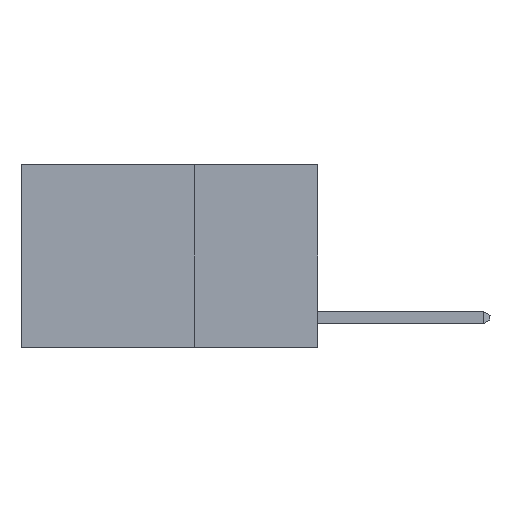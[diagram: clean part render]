
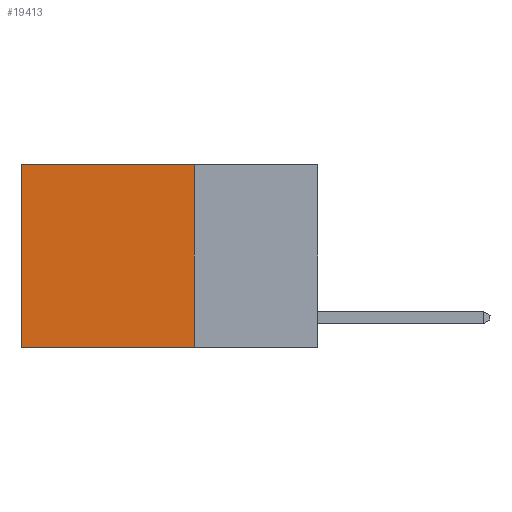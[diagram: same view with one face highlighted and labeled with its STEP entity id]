
A CAD part, left-side view. The second image highlights one B-rep face of the part: STEP entity #19413.
In plain terms, the highlighted planar face has unit normal (-1, 0, 0).
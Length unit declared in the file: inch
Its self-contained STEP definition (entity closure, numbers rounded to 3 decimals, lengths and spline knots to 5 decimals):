
#179 = ORIENTED_EDGE ( 'NONE', *, *, #16692, .T. ) ;
#418 = VECTOR ( 'NONE', #7568, 39.37008 ) ;
#4333 = PLANE ( 'NONE',  #17666 ) ;
#4831 = LINE ( 'NONE', #19243, #21026 ) ;
#5610 = CARTESIAN_POINT ( 'NONE',  ( 0.2625, 0.6, 0. ) ) ;
#5977 = DIRECTION ( 'NONE',  ( 0., 0., -1. ) ) ;
#6115 = DIRECTION ( 'NONE',  ( 0., 0., -1. ) ) ;
#6615 = ORIENTED_EDGE ( 'NONE', *, *, #10971, .F. ) ;
#6713 = VERTEX_POINT ( 'NONE', #22588 ) ;
#6715 = ORIENTED_EDGE ( 'NONE', *, *, #14011, .F. ) ;
#6773 = VECTOR ( 'NONE', #20077, 39.37008 ) ;
#7568 = DIRECTION ( 'NONE',  ( 0., 1., 0. ) ) ;
#9621 = LINE ( 'NONE', #16779, #17544 ) ;
#9947 = CARTESIAN_POINT ( 'NONE',  ( 0.2625, 0.25, 0. ) ) ;
#10971 = EDGE_CURVE ( 'NONE', #16279, #19286, #15123, .T. ) ;
#11966 = DIRECTION ( 'NONE',  ( 0., 0., -1. ) ) ;
#14011 = EDGE_CURVE ( 'NONE', #6713, #16279, #9621, .T. ) ;
#14102 = ORIENTED_EDGE ( 'NONE', *, *, #20391, .T. ) ;
#14498 = CARTESIAN_POINT ( 'NONE',  ( 0.2625, 0.25, -0.37 ) ) ;
#14810 = LINE ( 'NONE', #16474, #6773 ) ;
#15123 = LINE ( 'NONE', #16471, #418 ) ;
#16258 = VERTEX_POINT ( 'NONE', #5610 ) ;
#16279 = VERTEX_POINT ( 'NONE', #14498 ) ;
#16296 = CARTESIAN_POINT ( 'NONE',  ( 0.2625, 0.6, -0.37 ) ) ;
#16471 = CARTESIAN_POINT ( 'NONE',  ( 0.2625, 0.25, -0.37 ) ) ;
#16474 = CARTESIAN_POINT ( 'NONE',  ( 0.2625, 0.25, 0. ) ) ;
#16692 = EDGE_CURVE ( 'NONE', #6713, #16258, #14810, .T. ) ;
#16779 = CARTESIAN_POINT ( 'NONE',  ( 0.2625, 0.25, 0. ) ) ;
#16872 = FACE_OUTER_BOUND ( 'NONE', #18247, .T. ) ;
#17544 = VECTOR ( 'NONE', #6115, 39.37008 ) ;
#17666 = AXIS2_PLACEMENT_3D ( 'NONE', #9947, #22224, #5977 ) ;
#18247 = EDGE_LOOP ( 'NONE', ( #14102, #6615, #6715, #179 ) ) ;
#19243 = CARTESIAN_POINT ( 'NONE',  ( 0.2625, 0.6, 0. ) ) ;
#19286 = VERTEX_POINT ( 'NONE', #16296 ) ;
#19413 = ADVANCED_FACE ( 'NONE', ( #16872 ), #4333, .F. ) ;
#20077 = DIRECTION ( 'NONE',  ( 0., 1., 0. ) ) ;
#20391 = EDGE_CURVE ( 'NONE', #16258, #19286, #4831, .T. ) ;
#21026 = VECTOR ( 'NONE', #11966, 39.37008 ) ;
#22224 = DIRECTION ( 'NONE',  ( 1., 0., 0. ) ) ;
#22588 = CARTESIAN_POINT ( 'NONE',  ( 0.2625, 0.25, 0. ) ) ;
